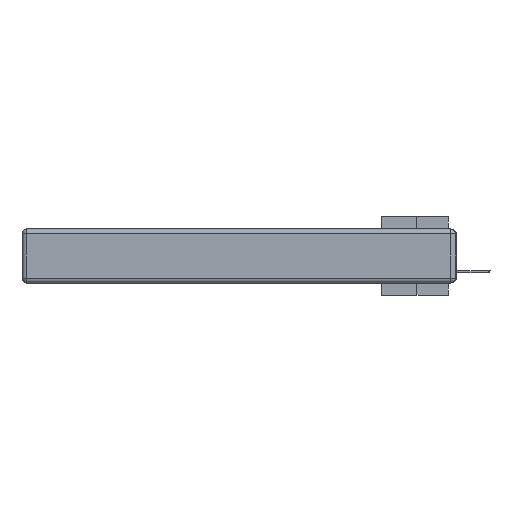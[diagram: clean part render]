
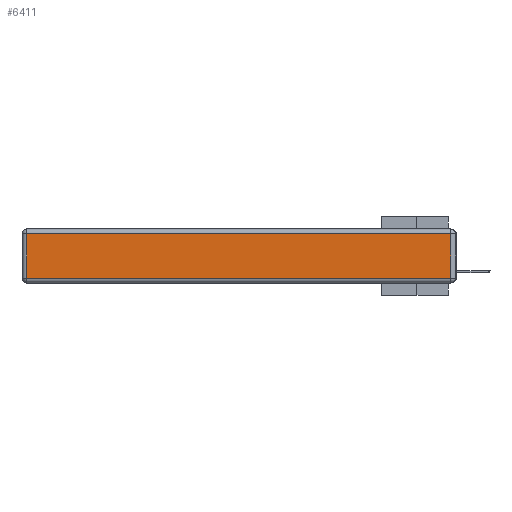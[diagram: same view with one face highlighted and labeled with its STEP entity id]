
A CAD part, left-side view. The second image highlights one B-rep face of the part: STEP entity #6411.
In plain terms, the highlighted planar face has unit normal (-1, 0, 0).
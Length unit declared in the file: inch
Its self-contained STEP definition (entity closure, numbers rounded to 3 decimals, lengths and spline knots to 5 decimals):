
#350 = VERTEX_POINT ( 'NONE', #17233 ) ;
#1075 = CARTESIAN_POINT ( 'NONE',  ( 0., 0., -0.343 ) ) ;
#1480 = VERTEX_POINT ( 'NONE', #29506 ) ;
#1544 = VECTOR ( 'NONE', #8228, 39.37008 ) ;
#2083 = LINE ( 'NONE', #24627, #17459 ) ;
#3037 = CARTESIAN_POINT ( 'NONE',  ( 0., 0., -0.313 ) ) ;
#4652 = DIRECTION ( 'NONE',  ( 0., 1., 0. ) ) ;
#6411 = ADVANCED_FACE ( 'NONE', ( #28838 ), #31439, .T. ) ;
#6451 = LINE ( 'NONE', #27369, #17684 ) ;
#6585 = DIRECTION ( 'NONE',  ( 0., 0., 1. ) ) ;
#8228 = DIRECTION ( 'NONE',  ( 0., -1., 0. ) ) ;
#9535 = AXIS2_PLACEMENT_3D ( 'NONE', #1075, #16026, #6585 ) ;
#11989 = DIRECTION ( 'NONE',  ( 0., 0., -1. ) ) ;
#12164 = DIRECTION ( 'NONE',  ( 0., 0., 1. ) ) ;
#12298 = EDGE_CURVE ( 'NONE', #26581, #1480, #14758, .T. ) ;
#12482 = CARTESIAN_POINT ( 'NONE',  ( 0., 0.03, -0.343 ) ) ;
#13416 = LINE ( 'NONE', #3037, #1544 ) ;
#14415 = VECTOR ( 'NONE', #12164, 39.37008 ) ;
#14514 = EDGE_LOOP ( 'NONE', ( #21876, #29368, #19833, #16404 ) ) ;
#14758 = LINE ( 'NONE', #12482, #14415 ) ;
#15298 = EDGE_CURVE ( 'NONE', #24227, #26581, #13416, .T. ) ;
#16026 = DIRECTION ( 'NONE',  ( -1., 0., 0. ) ) ;
#16404 = ORIENTED_EDGE ( 'NONE', *, *, #30821, .T. ) ;
#17233 = CARTESIAN_POINT ( 'NONE',  ( 0., 2.72, -0.03 ) ) ;
#17459 = VECTOR ( 'NONE', #11989, 39.37008 ) ;
#17684 = VECTOR ( 'NONE', #4652, 39.37008 ) ;
#19833 = ORIENTED_EDGE ( 'NONE', *, *, #20221, .T. ) ;
#20221 = EDGE_CURVE ( 'NONE', #1480, #350, #6451, .T. ) ;
#21876 = ORIENTED_EDGE ( 'NONE', *, *, #15298, .T. ) ;
#24227 = VERTEX_POINT ( 'NONE', #25205 ) ;
#24627 = CARTESIAN_POINT ( 'NONE',  ( 0., 2.72, -0.343 ) ) ;
#25205 = CARTESIAN_POINT ( 'NONE',  ( 0., 2.72, -0.313 ) ) ;
#26581 = VERTEX_POINT ( 'NONE', #29986 ) ;
#27369 = CARTESIAN_POINT ( 'NONE',  ( 0., 2.75, -0.03 ) ) ;
#28838 = FACE_OUTER_BOUND ( 'NONE', #14514, .T. ) ;
#29368 = ORIENTED_EDGE ( 'NONE', *, *, #12298, .T. ) ;
#29506 = CARTESIAN_POINT ( 'NONE',  ( 0., 0.03, -0.03 ) ) ;
#29986 = CARTESIAN_POINT ( 'NONE',  ( 0., 0.03, -0.313 ) ) ;
#30821 = EDGE_CURVE ( 'NONE', #350, #24227, #2083, .T. ) ;
#31439 = PLANE ( 'NONE',  #9535 ) ;
